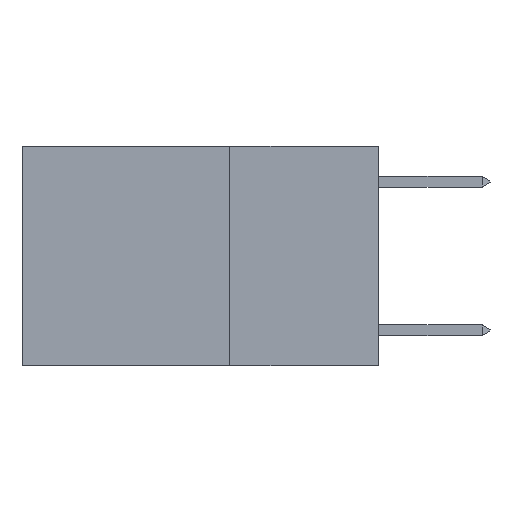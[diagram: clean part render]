
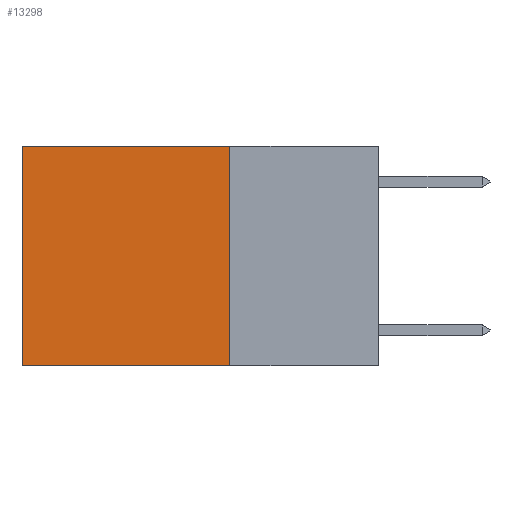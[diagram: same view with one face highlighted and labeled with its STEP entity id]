
A CAD part, left-side view. The second image highlights one B-rep face of the part: STEP entity #13298.
In plain terms, the highlighted planar face has unit normal (-1, 0, 0).
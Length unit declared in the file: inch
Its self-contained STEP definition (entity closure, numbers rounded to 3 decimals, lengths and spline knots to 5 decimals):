
#95 = CARTESIAN_POINT ( 'NONE',  ( 0.2625, 0.25, -0.37 ) ) ;
#414 = EDGE_CURVE ( 'NONE', #2167, #6344, #1698, .T. ) ;
#459 = LINE ( 'NONE', #3875, #14461 ) ;
#688 = LINE ( 'NONE', #5328, #10830 ) ;
#1468 = CARTESIAN_POINT ( 'NONE',  ( 0.2625, 0.25, 0. ) ) ;
#1698 = LINE ( 'NONE', #2705, #13357 ) ;
#1837 = CARTESIAN_POINT ( 'NONE',  ( 0.2625, 0.25, 0. ) ) ;
#1871 = EDGE_LOOP ( 'NONE', ( #13665, #10612, #3518, #14419 ) ) ;
#2060 = VERTEX_POINT ( 'NONE', #10299 ) ;
#2112 = AXIS2_PLACEMENT_3D ( 'NONE', #1837, #5049, #7494 ) ;
#2167 = VERTEX_POINT ( 'NONE', #1468 ) ;
#2705 = CARTESIAN_POINT ( 'NONE',  ( 0.2625, 0.25, 0. ) ) ;
#3264 = DIRECTION ( 'NONE',  ( 0., 0., -1. ) ) ;
#3518 = ORIENTED_EDGE ( 'NONE', *, *, #11288, .F. ) ;
#3587 = LINE ( 'NONE', #95, #9726 ) ;
#3875 = CARTESIAN_POINT ( 'NONE',  ( 0.2625, 0.25, 0. ) ) ;
#3993 = EDGE_CURVE ( 'NONE', #10585, #2060, #3587, .T. ) ;
#4057 = DIRECTION ( 'NONE',  ( 0., 1., 0. ) ) ;
#5049 = DIRECTION ( 'NONE',  ( 1., 0., 0. ) ) ;
#5328 = CARTESIAN_POINT ( 'NONE',  ( 0.2625, 0.6, 0. ) ) ;
#5441 = CARTESIAN_POINT ( 'NONE',  ( 0.2625, 0.25, -0.37 ) ) ;
#6344 = VERTEX_POINT ( 'NONE', #9801 ) ;
#7494 = DIRECTION ( 'NONE',  ( 0., 0., -1. ) ) ;
#9685 = DIRECTION ( 'NONE',  ( 0., 0., -1. ) ) ;
#9726 = VECTOR ( 'NONE', #10678, 39.37008 ) ;
#9801 = CARTESIAN_POINT ( 'NONE',  ( 0.2625, 0.6, 0. ) ) ;
#10299 = CARTESIAN_POINT ( 'NONE',  ( 0.2625, 0.6, -0.37 ) ) ;
#10585 = VERTEX_POINT ( 'NONE', #5441 ) ;
#10612 = ORIENTED_EDGE ( 'NONE', *, *, #3993, .F. ) ;
#10678 = DIRECTION ( 'NONE',  ( 0., 1., 0. ) ) ;
#10830 = VECTOR ( 'NONE', #3264, 39.37008 ) ;
#11288 = EDGE_CURVE ( 'NONE', #2167, #10585, #459, .T. ) ;
#11619 = EDGE_CURVE ( 'NONE', #6344, #2060, #688, .T. ) ;
#11970 = PLANE ( 'NONE',  #2112 ) ;
#13253 = FACE_OUTER_BOUND ( 'NONE', #1871, .T. ) ;
#13298 = ADVANCED_FACE ( 'NONE', ( #13253 ), #11970, .F. ) ;
#13357 = VECTOR ( 'NONE', #4057, 39.37008 ) ;
#13665 = ORIENTED_EDGE ( 'NONE', *, *, #11619, .T. ) ;
#14419 = ORIENTED_EDGE ( 'NONE', *, *, #414, .T. ) ;
#14461 = VECTOR ( 'NONE', #9685, 39.37008 ) ;
